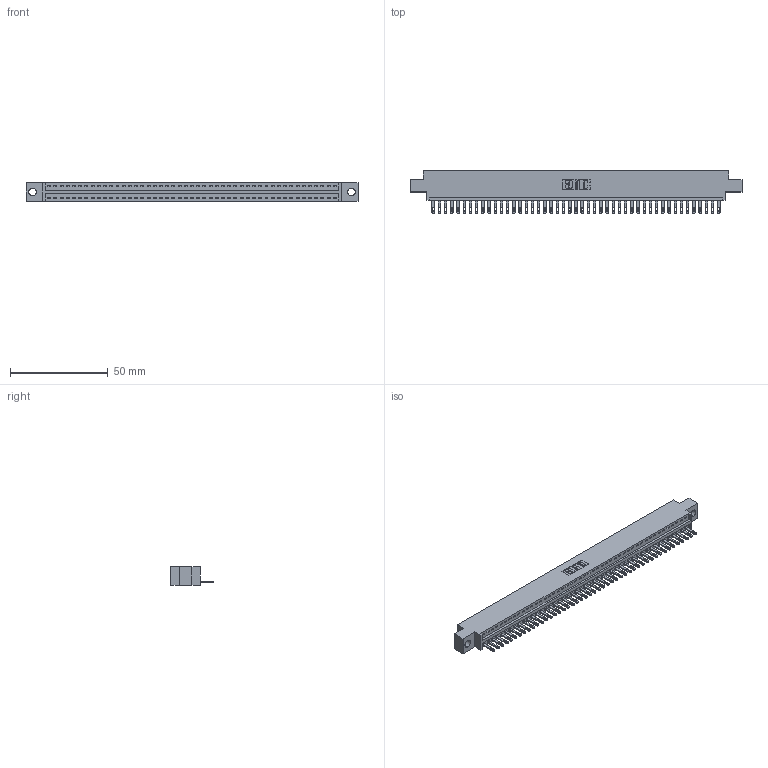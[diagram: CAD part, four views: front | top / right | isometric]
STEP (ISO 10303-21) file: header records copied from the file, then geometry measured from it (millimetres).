
FILE_DESCRIPTION (( 'STEP AP203' ), '1' );
FILE_NAME ('346-047-500-604.STEP', '2018-08-25T07:10:39', ( '' ), ( '' ), 'SwSTEP 2.0', 'SolidWorks 2016', '' );
FILE_SCHEMA (( 'CONFIG_CONTROL_DESIGN' ));
Length unit declared in the file: inch
Products named in the file (3): 345-292-001_345-293-100; 346-047-500-604; 346 Part_0.170 Offset - 0.156 Dia-TH
Assembly tree (48 placements, depth 2):
  346-047-500-604
    346 Part_0.170 Offset - 0.156 Dia-TH
    345-292-001_345-293-100  x47
Bounding box: 169.8 x 21.84 x 9.4 mm (x, y, z)
Volume: 16074.6 mm3; surface area: 20219.9 mm2
Topology: 48 solids, 48 shells, 2664 faces, 8237 edges, 5490 vertices
Faces by surface type: plane 1678, cylinder 986
Entity records: 28561 total; most frequent: CARTESIAN_POINT 4901, ORIENTED_EDGE 4882, DIRECTION 4319, EDGE_CURVE 2441, VECTOR 2117, LINE 2117, VERTEX_POINT 1626, AXIS2_PLACEMENT_3D 1101
